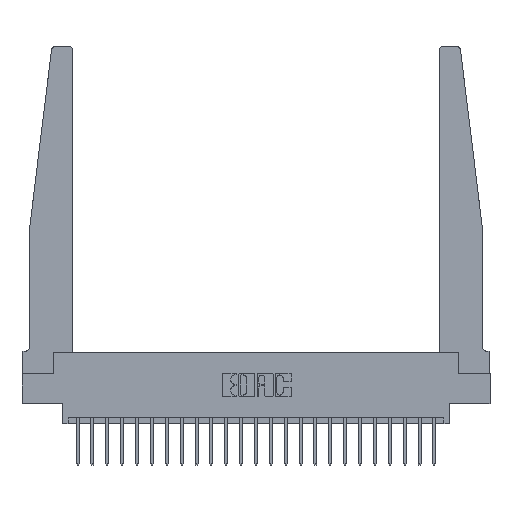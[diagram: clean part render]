
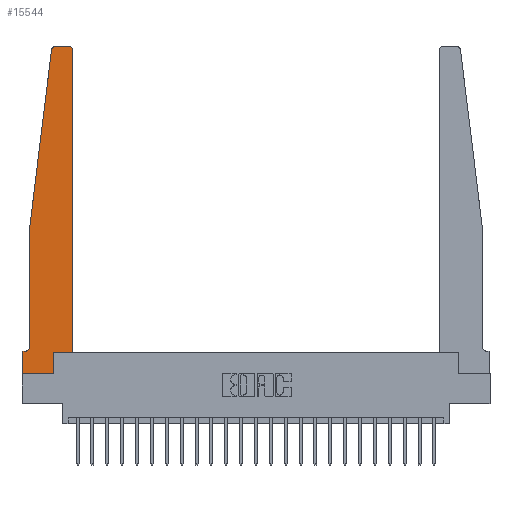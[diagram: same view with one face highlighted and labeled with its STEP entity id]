
A CAD part, top view. The second image highlights one B-rep face of the part: STEP entity #15544.
In plain terms, the highlighted planar face has unit normal (0, 0, 1).
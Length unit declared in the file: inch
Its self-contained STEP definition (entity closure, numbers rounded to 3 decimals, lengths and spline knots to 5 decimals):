
#291 = CARTESIAN_POINT ( 'NONE',  ( 0.27653, 2.72, 0.37 ) ) ;
#331 = CIRCLE ( 'NONE', #20762, 0.03 ) ;
#700 = ORIENTED_EDGE ( 'NONE', *, *, #2424, .T. ) ;
#763 = VECTOR ( 'NONE', #18329, 39.37008 ) ;
#1138 = CARTESIAN_POINT ( 'NONE',  ( 0.015, 0.1875, 0.37 ) ) ;
#1206 = CARTESIAN_POINT ( 'NONE',  ( 0., 0.1875, 0.37 ) ) ;
#1257 = VECTOR ( 'NONE', #14079, 39.37008 ) ;
#1352 = VERTEX_POINT ( 'NONE', #5621 ) ;
#1591 = CARTESIAN_POINT ( 'NONE',  ( 0.015, 0.2375, 0.37 ) ) ;
#1746 = CARTESIAN_POINT ( 'NONE',  ( 0.25, 2.75, 0.37 ) ) ;
#2108 = DIRECTION ( 'NONE',  ( 1., 0., 0. ) ) ;
#2167 = CIRCLE ( 'NONE', #22725, 0.05 ) ;
#2313 = VERTEX_POINT ( 'NONE', #13702 ) ;
#2424 = EDGE_CURVE ( 'NONE', #12202, #2313, #20613, .T. ) ;
#3234 = LINE ( 'NONE', #8181, #12367 ) ;
#3241 = LINE ( 'NONE', #5766, #12942 ) ;
#3273 = CARTESIAN_POINT ( 'NONE',  ( 0.065, 1.25, 0.37 ) ) ;
#3340 = EDGE_CURVE ( 'NONE', #14597, #20272, #14011, .T. ) ;
#3374 = CARTESIAN_POINT ( 'NONE',  ( 0.065, 0.2375, 0.37 ) ) ;
#3415 = DIRECTION ( 'NONE',  ( -1., 0., 0. ) ) ;
#3560 = EDGE_CURVE ( 'NONE', #5984, #14446, #331, .T. ) ;
#4247 = ORIENTED_EDGE ( 'NONE', *, *, #6463, .T. ) ;
#4272 = VERTEX_POINT ( 'NONE', #5309 ) ;
#4634 = CARTESIAN_POINT ( 'NONE',  ( 0.395, 2.72, 0.37 ) ) ;
#4780 = ORIENTED_EDGE ( 'NONE', *, *, #3340, .T. ) ;
#4849 = PLANE ( 'NONE',  #11506 ) ;
#5043 = LINE ( 'NONE', #7387, #763 ) ;
#5309 = CARTESIAN_POINT ( 'NONE',  ( 0.24675, 2.72367, 0.37 ) ) ;
#5621 = CARTESIAN_POINT ( 'NONE',  ( 0., 0., 0.37 ) ) ;
#5766 = CARTESIAN_POINT ( 'NONE',  ( 0.425, 0.18, 0.37 ) ) ;
#5866 = DIRECTION ( 'NONE',  ( -1., 0., 0. ) ) ;
#5984 = VERTEX_POINT ( 'NONE', #7880 ) ;
#6122 = LINE ( 'NONE', #10436, #1257 ) ;
#6248 = ORIENTED_EDGE ( 'NONE', *, *, #17118, .T. ) ;
#6463 = EDGE_CURVE ( 'NONE', #21205, #4272, #14154, .T. ) ;
#6507 = DIRECTION ( 'NONE',  ( 1., 0., 0. ) ) ;
#7038 = CARTESIAN_POINT ( 'NONE',  ( 0.2605, 0., 0.37 ) ) ;
#7387 = CARTESIAN_POINT ( 'NONE',  ( 0.065, 1.25, 0.37 ) ) ;
#7568 = CARTESIAN_POINT ( 'NONE',  ( 0.2605, 0.18, 0.37 ) ) ;
#7687 = DIRECTION ( 'NONE',  ( 0., -1., 0. ) ) ;
#7880 = CARTESIAN_POINT ( 'NONE',  ( 0.425, 2.72, 0.37 ) ) ;
#8090 = EDGE_CURVE ( 'NONE', #12434, #12202, #19548, .T. ) ;
#8181 = CARTESIAN_POINT ( 'NONE',  ( 0., 0., 0.37 ) ) ;
#8533 = CARTESIAN_POINT ( 'NONE',  ( 0., 0.1875, 0.37 ) ) ;
#9023 = DIRECTION ( 'NONE',  ( -1., 0., 0. ) ) ;
#9396 = DIRECTION ( 'NONE',  ( 0., 1., 0. ) ) ;
#9752 = VECTOR ( 'NONE', #5866, 39.37008 ) ;
#10003 = VERTEX_POINT ( 'NONE', #3374 ) ;
#10373 = DIRECTION ( 'NONE',  ( 1., 0., 0. ) ) ;
#10436 = CARTESIAN_POINT ( 'NONE',  ( 0., 0., 0.37 ) ) ;
#10445 = CARTESIAN_POINT ( 'NONE',  ( 0.425, 0.18, 0.37 ) ) ;
#10658 = VERTEX_POINT ( 'NONE', #3273 ) ;
#10940 = VECTOR ( 'NONE', #21315, 39.37008 ) ;
#11328 = ORIENTED_EDGE ( 'NONE', *, *, #14184, .T. ) ;
#11506 = AXIS2_PLACEMENT_3D ( 'NONE', #8533, #21238, #10373 ) ;
#11520 = CARTESIAN_POINT ( 'NONE',  ( 0.395, 2.75, 0.37 ) ) ;
#12202 = VERTEX_POINT ( 'NONE', #16793 ) ;
#12298 = ORIENTED_EDGE ( 'NONE', *, *, #8090, .T. ) ;
#12367 = VECTOR ( 'NONE', #13667, 39.37008 ) ;
#12434 = VERTEX_POINT ( 'NONE', #7038 ) ;
#12942 = VECTOR ( 'NONE', #18552, 39.37008 ) ;
#13038 = DIRECTION ( 'NONE',  ( 0., 0., 1. ) ) ;
#13270 = ORIENTED_EDGE ( 'NONE', *, *, #19841, .T. ) ;
#13423 = LINE ( 'NONE', #1746, #18298 ) ;
#13472 = FACE_OUTER_BOUND ( 'NONE', #17000, .T. ) ;
#13604 = EDGE_CURVE ( 'NONE', #10003, #14597, #2167, .T. ) ;
#13667 = DIRECTION ( 'NONE',  ( 0., -1., 0. ) ) ;
#13702 = CARTESIAN_POINT ( 'NONE',  ( 0.425, 0.18, 0.37 ) ) ;
#14011 = LINE ( 'NONE', #14955, #9752 ) ;
#14079 = DIRECTION ( 'NONE',  ( 1., 0., 0. ) ) ;
#14154 = CIRCLE ( 'NONE', #19772, 0.03 ) ;
#14184 = EDGE_CURVE ( 'NONE', #1352, #12434, #6122, .T. ) ;
#14344 = DIRECTION ( 'NONE',  ( 0., 0., -1. ) ) ;
#14446 = VERTEX_POINT ( 'NONE', #11520 ) ;
#14597 = VERTEX_POINT ( 'NONE', #1138 ) ;
#14689 = VECTOR ( 'NONE', #9396, 39.37008 ) ;
#14831 = EDGE_CURVE ( 'NONE', #2313, #5984, #3241, .T. ) ;
#14955 = CARTESIAN_POINT ( 'NONE',  ( 0.065, 0.1875, 0.37 ) ) ;
#15544 = ADVANCED_FACE ( 'NONE', ( #13472 ), #4849, .T. ) ;
#16793 = CARTESIAN_POINT ( 'NONE',  ( 0.2605, 0.18, 0.37 ) ) ;
#16897 = VECTOR ( 'NONE', #7687, 39.37008 ) ;
#17000 = EDGE_LOOP ( 'NONE', ( #20911, #4247, #13270, #6248, #23400, #4780, #17492, #11328, #12298, #700, #19710, #21560 ) ) ;
#17118 = EDGE_CURVE ( 'NONE', #10658, #10003, #21096, .T. ) ;
#17436 = DIRECTION ( 'NONE',  ( 0., 0., 1. ) ) ;
#17492 = ORIENTED_EDGE ( 'NONE', *, *, #21944, .T. ) ;
#18298 = VECTOR ( 'NONE', #9023, 39.37008 ) ;
#18329 = DIRECTION ( 'NONE',  ( -0.122, -0.992, 0. ) ) ;
#18552 = DIRECTION ( 'NONE',  ( 0., 1., 0. ) ) ;
#18620 = CARTESIAN_POINT ( 'NONE',  ( 0.065, 1.25, 0.37 ) ) ;
#19548 = LINE ( 'NONE', #7568, #14689 ) ;
#19710 = ORIENTED_EDGE ( 'NONE', *, *, #14831, .T. ) ;
#19772 = AXIS2_PLACEMENT_3D ( 'NONE', #291, #13038, #2108 ) ;
#19841 = EDGE_CURVE ( 'NONE', #4272, #10658, #5043, .T. ) ;
#20229 = CARTESIAN_POINT ( 'NONE',  ( 0.27653, 2.75, 0.37 ) ) ;
#20272 = VERTEX_POINT ( 'NONE', #1206 ) ;
#20613 = LINE ( 'NONE', #10445, #10940 ) ;
#20762 = AXIS2_PLACEMENT_3D ( 'NONE', #4634, #17436, #6507 ) ;
#20911 = ORIENTED_EDGE ( 'NONE', *, *, #22800, .T. ) ;
#21096 = LINE ( 'NONE', #18620, #16897 ) ;
#21205 = VERTEX_POINT ( 'NONE', #20229 ) ;
#21238 = DIRECTION ( 'NONE',  ( 0., 0., 1. ) ) ;
#21315 = DIRECTION ( 'NONE',  ( 1., 0., 0. ) ) ;
#21560 = ORIENTED_EDGE ( 'NONE', *, *, #3560, .T. ) ;
#21944 = EDGE_CURVE ( 'NONE', #20272, #1352, #3234, .T. ) ;
#22725 = AXIS2_PLACEMENT_3D ( 'NONE', #1591, #14344, #3415 ) ;
#22800 = EDGE_CURVE ( 'NONE', #14446, #21205, #13423, .T. ) ;
#23400 = ORIENTED_EDGE ( 'NONE', *, *, #13604, .T. ) ;
